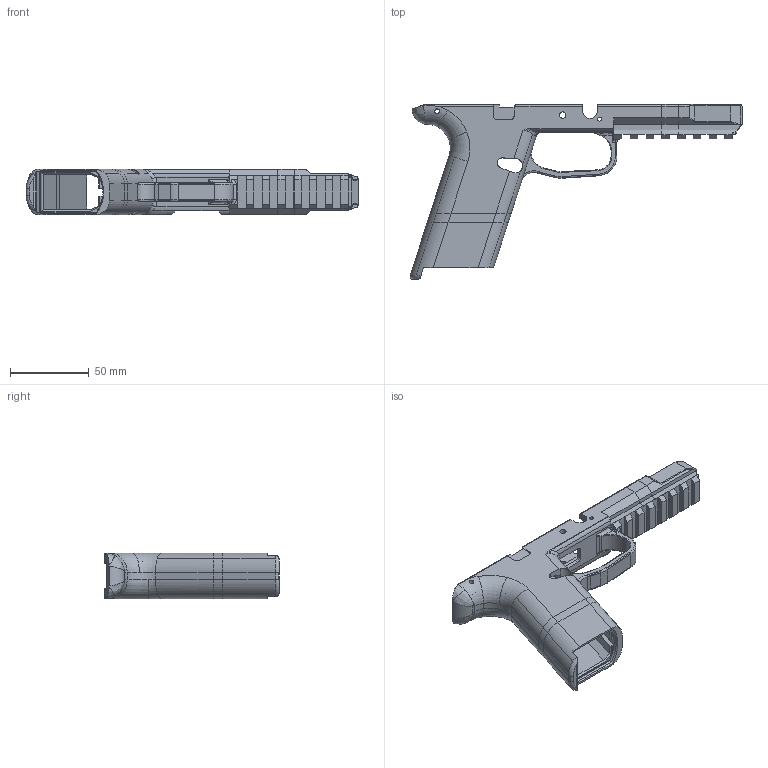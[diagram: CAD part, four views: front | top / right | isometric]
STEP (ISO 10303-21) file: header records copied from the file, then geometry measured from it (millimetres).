
FILE_DESCRIPTION (( 'STEP AP203' ), '1' );
FILE_NAME ('Longslide_yes_beavertale.STEP', '2021-05-30T00:56:31', ( '' ), ( '' ), 'SwSTEP 2.0', 'SolidWorks 2020', '' );
FILE_SCHEMA (( 'CONFIG_CONTROL_DESIGN' ));
Length unit declared in the file: millimetre
Products named in the file (1): Longslide_yes_beavertale
Bounding box: 210.6 x 110.97 x 29 mm (x, y, z)
Volume: 92680.4 mm3; surface area: 52007.5 mm2
Topology: 5 solids, 5 shells, 578 faces, 1628 edges, 1046 vertices
Faces by surface type: plane 299, cylinder 205, torus 36, bspline 32, cone 6
Entity records: 20156 total; most frequent: CARTESIAN_POINT 5766, ORIENTED_EDGE 3248, DIRECTION 2703, EDGE_CURVE 1624, VERTEX_POINT 1046, LINE 1025, VECTOR 1025, AXIS2_PLACEMENT_3D 839
